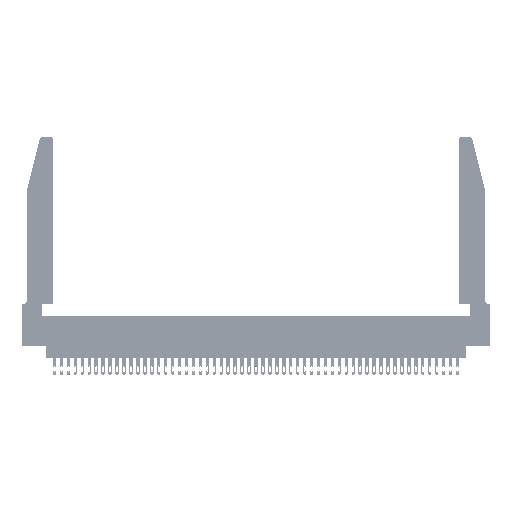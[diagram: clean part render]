
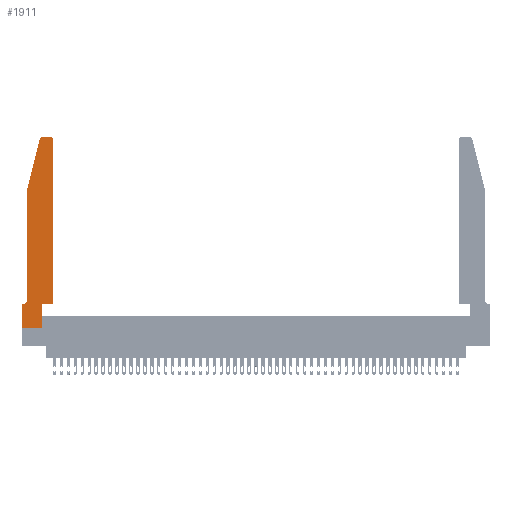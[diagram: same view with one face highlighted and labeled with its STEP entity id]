
A CAD part, top view. The second image highlights one B-rep face of the part: STEP entity #1911.
In plain terms, the highlighted planar face has unit normal (0, 0, 1).
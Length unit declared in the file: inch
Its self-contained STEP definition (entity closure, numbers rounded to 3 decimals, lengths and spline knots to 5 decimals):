
#492 = DIRECTION ( 'NONE',  ( 0., 0., 1. ) ) ;
#765 = LINE ( 'NONE', #47830, #5522 ) ;
#1141 = VECTOR ( 'NONE', #11594, 39.37008 ) ;
#1653 = LINE ( 'NONE', #19113, #16470 ) ;
#1911 = ADVANCED_FACE ( 'NONE', ( #33238 ), #13924, .T. ) ;
#2218 = ORIENTED_EDGE ( 'NONE', *, *, #15167, .T. ) ;
#2842 = EDGE_CURVE ( 'NONE', #11180, #37859, #12570, .T. ) ;
#4108 = ORIENTED_EDGE ( 'NONE', *, *, #19035, .T. ) ;
#4457 = EDGE_CURVE ( 'NONE', #27892, #48066, #32006, .T. ) ;
#4579 = CARTESIAN_POINT ( 'NONE',  ( 0.0755, 0.42, 0.37 ) ) ;
#5522 = VECTOR ( 'NONE', #39770, 39.37008 ) ;
#5745 = VERTEX_POINT ( 'NONE', #19603 ) ;
#6031 = ORIENTED_EDGE ( 'NONE', *, *, #39348, .T. ) ;
#6129 = AXIS2_PLACEMENT_3D ( 'NONE', #9663, #17265, #44212 ) ;
#6133 = DIRECTION ( 'NONE',  ( 0., 0., 1. ) ) ;
#6591 = CIRCLE ( 'NONE', #41407, 0.03 ) ;
#7707 = VERTEX_POINT ( 'NONE', #48059 ) ;
#8857 = LINE ( 'NONE', #18883, #1141 ) ;
#8859 = DIRECTION ( 'NONE',  ( 0., -1., 0. ) ) ;
#9663 = CARTESIAN_POINT ( 'NONE',  ( 0.0055, 0.42, 0.37 ) ) ;
#10499 = CARTESIAN_POINT ( 'NONE',  ( 0.0055, 0.35, 0.37 ) ) ;
#11180 = VERTEX_POINT ( 'NONE', #20121 ) ;
#11594 = DIRECTION ( 'NONE',  ( -0.239, -0.971, 0. ) ) ;
#11939 = DIRECTION ( 'NONE',  ( 1., 0., 0. ) ) ;
#12570 = LINE ( 'NONE', #38393, #23747 ) ;
#13924 = PLANE ( 'NONE',  #43997 ) ;
#14091 = VECTOR ( 'NONE', #30847, 39.37008 ) ;
#14400 = CARTESIAN_POINT ( 'NONE',  ( 0.0755, 0.35, 0.37 ) ) ;
#15167 = EDGE_CURVE ( 'NONE', #48066, #7707, #31104, .T. ) ;
#16463 = VECTOR ( 'NONE', #29524, 39.37008 ) ;
#16470 = VECTOR ( 'NONE', #38313, 39.37008 ) ;
#17265 = DIRECTION ( 'NONE',  ( 0., 0., -1. ) ) ;
#18233 = VECTOR ( 'NONE', #8859, 39.37008 ) ;
#18883 = CARTESIAN_POINT ( 'NONE',  ( 0.0755, 2., 0.37 ) ) ;
#19035 = EDGE_CURVE ( 'NONE', #20390, #27580, #8857, .T. ) ;
#19113 = CARTESIAN_POINT ( 'NONE',  ( 0.2865, 0.35, 0.37 ) ) ;
#19603 = CARTESIAN_POINT ( 'NONE',  ( 0., 0.35, 0.37 ) ) ;
#20121 = CARTESIAN_POINT ( 'NONE',  ( 0.2865, 0.35, 0.37 ) ) ;
#20390 = VERTEX_POINT ( 'NONE', #27428 ) ;
#22223 = CARTESIAN_POINT ( 'NONE',  ( 0., 0., 0.37 ) ) ;
#22331 = LINE ( 'NONE', #46035, #18233 ) ;
#22974 = DIRECTION ( 'NONE',  ( 0., 1., 0. ) ) ;
#23747 = VECTOR ( 'NONE', #38228, 39.37008 ) ;
#23951 = CARTESIAN_POINT ( 'NONE',  ( 0.4505, 2.72, 0.37 ) ) ;
#25366 = EDGE_CURVE ( 'NONE', #46510, #31804, #765, .T. ) ;
#25873 = CARTESIAN_POINT ( 'NONE',  ( 0.2605, 2.75, 0.37 ) ) ;
#26033 = CARTESIAN_POINT ( 'NONE',  ( 0.2865, 0., 0.37 ) ) ;
#26434 = LINE ( 'NONE', #45956, #14091 ) ;
#26718 = CARTESIAN_POINT ( 'NONE',  ( 0.0755, 2., 0.37 ) ) ;
#27428 = CARTESIAN_POINT ( 'NONE',  ( 0.25487, 2.72718, 0.37 ) ) ;
#27580 = VERTEX_POINT ( 'NONE', #26718 ) ;
#27674 = EDGE_CURVE ( 'NONE', #7707, #20390, #6591, .T. ) ;
#27892 = VERTEX_POINT ( 'NONE', #23951 ) ;
#28164 = LINE ( 'NONE', #45329, #47591 ) ;
#28428 = VERTEX_POINT ( 'NONE', #4579 ) ;
#29524 = DIRECTION ( 'NONE',  ( -1., 0., 0. ) ) ;
#30847 = DIRECTION ( 'NONE',  ( 0., -1., 0. ) ) ;
#31104 = LINE ( 'NONE', #25873, #39905 ) ;
#31804 = VERTEX_POINT ( 'NONE', #26033 ) ;
#32006 = CIRCLE ( 'NONE', #36502, 0.03 ) ;
#33016 = EDGE_CURVE ( 'NONE', #37859, #27892, #28164, .T. ) ;
#33238 = FACE_OUTER_BOUND ( 'NONE', #44879, .T. ) ;
#33847 = ORIENTED_EDGE ( 'NONE', *, *, #45191, .T. ) ;
#34705 = LINE ( 'NONE', #14400, #16463 ) ;
#35402 = ORIENTED_EDGE ( 'NONE', *, *, #41453, .T. ) ;
#36502 = AXIS2_PLACEMENT_3D ( 'NONE', #39269, #46364, #43223 ) ;
#37248 = ORIENTED_EDGE ( 'NONE', *, *, #39236, .T. ) ;
#37469 = CIRCLE ( 'NONE', #6129, 0.07 ) ;
#37859 = VERTEX_POINT ( 'NONE', #40557 ) ;
#37909 = ORIENTED_EDGE ( 'NONE', *, *, #2842, .T. ) ;
#37929 = ORIENTED_EDGE ( 'NONE', *, *, #25366, .T. ) ;
#38228 = DIRECTION ( 'NONE',  ( 1., 0., 0. ) ) ;
#38313 = DIRECTION ( 'NONE',  ( 0., 1., 0. ) ) ;
#38393 = CARTESIAN_POINT ( 'NONE',  ( 0.4505, 0.35, 0.37 ) ) ;
#38889 = ORIENTED_EDGE ( 'NONE', *, *, #45073, .T. ) ;
#39236 = EDGE_CURVE ( 'NONE', #31804, #11180, #1653, .T. ) ;
#39269 = CARTESIAN_POINT ( 'NONE',  ( 0.4205, 2.72, 0.37 ) ) ;
#39348 = EDGE_CURVE ( 'NONE', #27580, #28428, #22331, .T. ) ;
#39475 = ORIENTED_EDGE ( 'NONE', *, *, #4457, .T. ) ;
#39770 = DIRECTION ( 'NONE',  ( 1., 0., 0. ) ) ;
#39905 = VECTOR ( 'NONE', #44943, 39.37008 ) ;
#40557 = CARTESIAN_POINT ( 'NONE',  ( 0.4505, 0.35, 0.37 ) ) ;
#41407 = AXIS2_PLACEMENT_3D ( 'NONE', #45831, #492, #11939 ) ;
#41453 = EDGE_CURVE ( 'NONE', #28428, #46351, #37469, .T. ) ;
#42007 = ORIENTED_EDGE ( 'NONE', *, *, #27674, .T. ) ;
#43223 = DIRECTION ( 'NONE',  ( 1., 0., 0. ) ) ;
#43374 = CARTESIAN_POINT ( 'NONE',  ( 0., 0.35, 0.37 ) ) ;
#43691 = DIRECTION ( 'NONE',  ( 1., 0., 0. ) ) ;
#43997 = AXIS2_PLACEMENT_3D ( 'NONE', #43374, #6133, #43691 ) ;
#44212 = DIRECTION ( 'NONE',  ( -1., 0., 0. ) ) ;
#44879 = EDGE_LOOP ( 'NONE', ( #2218, #42007, #4108, #6031, #35402, #33847, #38889, #37929, #37248, #37909, #47560, #39475 ) ) ;
#44943 = DIRECTION ( 'NONE',  ( -1., 0., 0. ) ) ;
#45073 = EDGE_CURVE ( 'NONE', #5745, #46510, #26434, .T. ) ;
#45191 = EDGE_CURVE ( 'NONE', #46351, #5745, #34705, .T. ) ;
#45329 = CARTESIAN_POINT ( 'NONE',  ( 0.4505, 0.35, 0.37 ) ) ;
#45740 = CARTESIAN_POINT ( 'NONE',  ( 0.4205, 2.75, 0.37 ) ) ;
#45831 = CARTESIAN_POINT ( 'NONE',  ( 0.284, 2.72, 0.37 ) ) ;
#45956 = CARTESIAN_POINT ( 'NONE',  ( 0., 0., 0.37 ) ) ;
#46035 = CARTESIAN_POINT ( 'NONE',  ( 0.0755, 2., 0.37 ) ) ;
#46351 = VERTEX_POINT ( 'NONE', #10499 ) ;
#46364 = DIRECTION ( 'NONE',  ( 0., 0., 1. ) ) ;
#46510 = VERTEX_POINT ( 'NONE', #22223 ) ;
#47560 = ORIENTED_EDGE ( 'NONE', *, *, #33016, .T. ) ;
#47591 = VECTOR ( 'NONE', #22974, 39.37008 ) ;
#47830 = CARTESIAN_POINT ( 'NONE',  ( 0., 0., 0.37 ) ) ;
#48059 = CARTESIAN_POINT ( 'NONE',  ( 0.284, 2.75, 0.37 ) ) ;
#48066 = VERTEX_POINT ( 'NONE', #45740 ) ;
